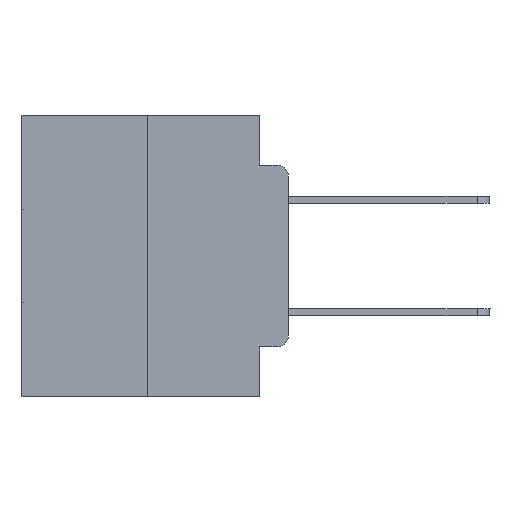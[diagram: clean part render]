
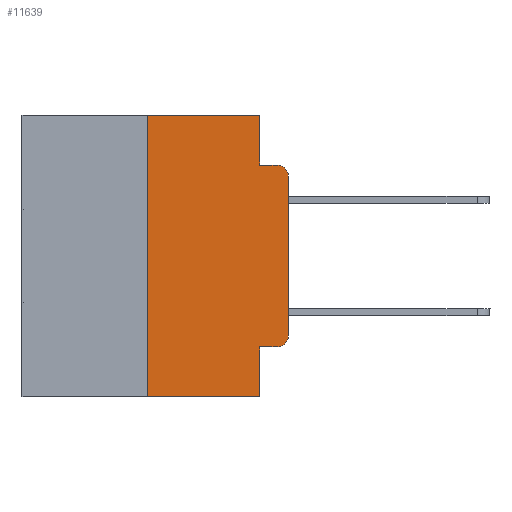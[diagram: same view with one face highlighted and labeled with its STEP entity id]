
A CAD part, left-side view. The second image highlights one B-rep face of the part: STEP entity #11639.
In plain terms, the highlighted planar face has unit normal (-1, 0, 0).
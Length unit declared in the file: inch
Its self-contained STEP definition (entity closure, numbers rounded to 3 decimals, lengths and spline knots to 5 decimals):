
#547 = DIRECTION ( 'NONE',  ( 0., 0., -1. ) ) ;
#571 = PLANE ( 'NONE',  #29308 ) ;
#680 = VERTEX_POINT ( 'NONE', #17295 ) ;
#985 = AXIS2_PLACEMENT_3D ( 'NONE', #16138, #11582, #20265 ) ;
#1374 = VERTEX_POINT ( 'NONE', #26192 ) ;
#2661 = DIRECTION ( 'NONE',  ( 0., 0., 1. ) ) ;
#2776 = DIRECTION ( 'NONE',  ( 0., -1., 0. ) ) ;
#3231 = CARTESIAN_POINT ( 'NONE',  ( 0., 0.051, -0.4115 ) ) ;
#3254 = LINE ( 'NONE', #12828, #20458 ) ;
#3311 = VECTOR ( 'NONE', #15803, 39.37008 ) ;
#3721 = VECTOR ( 'NONE', #3754, 39.37008 ) ;
#3754 = DIRECTION ( 'NONE',  ( 0., 0., 1. ) ) ;
#3851 = EDGE_LOOP ( 'NONE', ( #18351, #24800, #5205, #29899, #27401, #12977, #25872, #20303, #7815, #15926 ) ) ;
#4123 = VERTEX_POINT ( 'NONE', #16301 ) ;
#4879 = DIRECTION ( 'NONE',  ( -1., 0., 0. ) ) ;
#5125 = CARTESIAN_POINT ( 'NONE',  ( 0., 0.051, 0. ) ) ;
#5205 = ORIENTED_EDGE ( 'NONE', *, *, #28572, .F. ) ;
#5280 = DIRECTION ( 'NONE',  ( 0., 0., -1. ) ) ;
#5932 = DIRECTION ( 'NONE',  ( 0., -1., 0. ) ) ;
#5990 = VECTOR ( 'NONE', #5932, 39.37008 ) ;
#6199 = VERTEX_POINT ( 'NONE', #11874 ) ;
#6378 = EDGE_CURVE ( 'NONE', #18625, #29133, #19135, .T. ) ;
#7080 = LINE ( 'NONE', #27958, #9045 ) ;
#7168 = CARTESIAN_POINT ( 'NONE',  ( 0., 0.02, -0.1085 ) ) ;
#7350 = EDGE_CURVE ( 'NONE', #680, #1374, #24651, .T. ) ;
#7815 = ORIENTED_EDGE ( 'NONE', *, *, #20280, .T. ) ;
#8460 = CARTESIAN_POINT ( 'NONE',  ( 0., 0.051, -0.4115 ) ) ;
#8472 = EDGE_CURVE ( 'NONE', #1374, #18625, #16601, .T. ) ;
#9045 = VECTOR ( 'NONE', #2661, 39.37008 ) ;
#9508 = EDGE_CURVE ( 'NONE', #680, #15481, #3254, .T. ) ;
#9839 = CARTESIAN_POINT ( 'NONE',  ( 0., 0.473, 0. ) ) ;
#9898 = CARTESIAN_POINT ( 'NONE',  ( 0., 0.473, 0. ) ) ;
#9986 = FACE_OUTER_BOUND ( 'NONE', #3851, .T. ) ;
#10548 = DIRECTION ( 'NONE',  ( 0., -1., 0. ) ) ;
#10600 = VECTOR ( 'NONE', #2776, 39.37008 ) ;
#10700 = AXIS2_PLACEMENT_3D ( 'NONE', #7168, #4879, #14446 ) ;
#11465 = VECTOR ( 'NONE', #547, 39.37008 ) ;
#11582 = DIRECTION ( 'NONE',  ( -1., 0., 0. ) ) ;
#11639 = ADVANCED_FACE ( 'NONE', ( #9986 ), #571, .F. ) ;
#11874 = CARTESIAN_POINT ( 'NONE',  ( 0., 0.02, -0.0885 ) ) ;
#12054 = CARTESIAN_POINT ( 'NONE',  ( 0., 0., -0.3915 ) ) ;
#12828 = CARTESIAN_POINT ( 'NONE',  ( 0., 0.473, -0.5 ) ) ;
#12841 = EDGE_CURVE ( 'NONE', #29889, #6199, #19932, .T. ) ;
#12977 = ORIENTED_EDGE ( 'NONE', *, *, #7350, .F. ) ;
#13868 = DIRECTION ( 'NONE',  ( 0., -1., 0. ) ) ;
#14446 = DIRECTION ( 'NONE',  ( 0., 0., -1. ) ) ;
#15348 = LINE ( 'NONE', #24687, #5990 ) ;
#15470 = EDGE_CURVE ( 'NONE', #18908, #15481, #20562, .T. ) ;
#15481 = VERTEX_POINT ( 'NONE', #25135 ) ;
#15803 = DIRECTION ( 'NONE',  ( 0., 0., -1. ) ) ;
#15926 = ORIENTED_EDGE ( 'NONE', *, *, #23985, .T. ) ;
#16138 = CARTESIAN_POINT ( 'NONE',  ( 0., 0.02, -0.3915 ) ) ;
#16301 = CARTESIAN_POINT ( 'NONE',  ( 0., 0.02, -0.4115 ) ) ;
#16601 = LINE ( 'NONE', #9898, #22331 ) ;
#17295 = CARTESIAN_POINT ( 'NONE',  ( 0., 0.25, -0.5 ) ) ;
#17734 = EDGE_CURVE ( 'NONE', #20294, #29889, #7080, .T. ) ;
#17914 = CARTESIAN_POINT ( 'NONE',  ( 0., 0.051, -0.0885 ) ) ;
#18351 = ORIENTED_EDGE ( 'NONE', *, *, #17734, .T. ) ;
#18625 = VERTEX_POINT ( 'NONE', #5125 ) ;
#18908 = VERTEX_POINT ( 'NONE', #8460 ) ;
#18985 = CARTESIAN_POINT ( 'NONE',  ( 0., 0.051, 0. ) ) ;
#19135 = LINE ( 'NONE', #18985, #11465 ) ;
#19160 = DIRECTION ( 'NONE',  ( 1., 0., 0. ) ) ;
#19229 = LINE ( 'NONE', #3231, #10600 ) ;
#19497 = CARTESIAN_POINT ( 'NONE',  ( 0., 0., -0.1085 ) ) ;
#19932 = CIRCLE ( 'NONE', #10700, 0.02 ) ;
#20200 = CARTESIAN_POINT ( 'NONE',  ( 0., 0.25, 0. ) ) ;
#20265 = DIRECTION ( 'NONE',  ( 0., 0., -1. ) ) ;
#20280 = EDGE_CURVE ( 'NONE', #18908, #4123, #19229, .T. ) ;
#20294 = VERTEX_POINT ( 'NONE', #12054 ) ;
#20303 = ORIENTED_EDGE ( 'NONE', *, *, #15470, .F. ) ;
#20400 = CARTESIAN_POINT ( 'NONE',  ( 0., 0.051, 0. ) ) ;
#20458 = VECTOR ( 'NONE', #10548, 39.37008 ) ;
#20562 = LINE ( 'NONE', #20400, #3311 ) ;
#22331 = VECTOR ( 'NONE', #13868, 39.37008 ) ;
#23985 = EDGE_CURVE ( 'NONE', #4123, #20294, #28256, .T. ) ;
#24651 = LINE ( 'NONE', #20200, #3721 ) ;
#24687 = CARTESIAN_POINT ( 'NONE',  ( 0., 0.051, -0.0885 ) ) ;
#24800 = ORIENTED_EDGE ( 'NONE', *, *, #12841, .T. ) ;
#25135 = CARTESIAN_POINT ( 'NONE',  ( 0., 0.051, -0.5 ) ) ;
#25872 = ORIENTED_EDGE ( 'NONE', *, *, #9508, .T. ) ;
#26192 = CARTESIAN_POINT ( 'NONE',  ( 0., 0.25, 0. ) ) ;
#27401 = ORIENTED_EDGE ( 'NONE', *, *, #8472, .F. ) ;
#27958 = CARTESIAN_POINT ( 'NONE',  ( 0., 0., 0. ) ) ;
#28256 = CIRCLE ( 'NONE', #985, 0.02 ) ;
#28572 = EDGE_CURVE ( 'NONE', #29133, #6199, #15348, .T. ) ;
#29133 = VERTEX_POINT ( 'NONE', #17914 ) ;
#29308 = AXIS2_PLACEMENT_3D ( 'NONE', #9839, #19160, #5280 ) ;
#29889 = VERTEX_POINT ( 'NONE', #19497 ) ;
#29899 = ORIENTED_EDGE ( 'NONE', *, *, #6378, .F. ) ;
